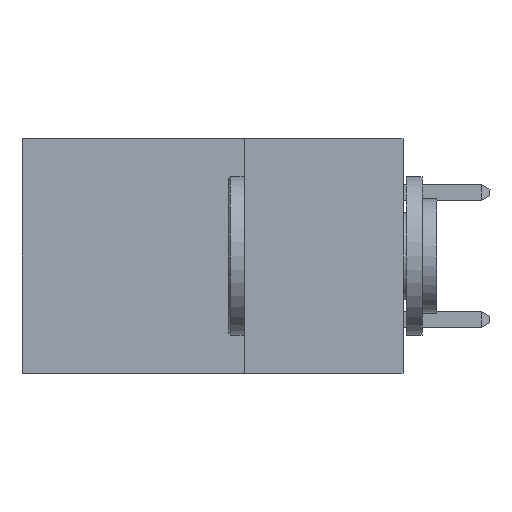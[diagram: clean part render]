
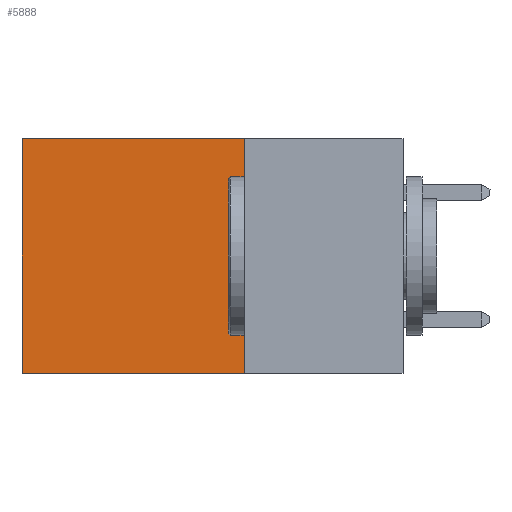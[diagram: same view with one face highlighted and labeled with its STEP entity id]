
A CAD part, left-side view. The second image highlights one B-rep face of the part: STEP entity #5888.
In plain terms, the highlighted planar face has unit normal (-1, 0, 0).
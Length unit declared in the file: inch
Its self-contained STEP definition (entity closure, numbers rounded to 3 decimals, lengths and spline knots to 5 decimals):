
#32 = VECTOR ( 'NONE', #170, 39.37008 ) ;
#118 = CARTESIAN_POINT ( 'NONE',  ( 0.2875, 0.25, -0.37 ) ) ;
#170 = DIRECTION ( 'NONE',  ( 0., 1., 0. ) ) ;
#578 = LINE ( 'NONE', #11281, #11457 ) ;
#1459 = EDGE_CURVE ( 'NONE', #9048, #6883, #3397, .T. ) ;
#2015 = EDGE_CURVE ( 'NONE', #9216, #11990, #4207, .T. ) ;
#2278 = DIRECTION ( 'NONE',  ( 1., 0., 0. ) ) ;
#2710 = ORIENTED_EDGE ( 'NONE', *, *, #3335, .F. ) ;
#3250 = CARTESIAN_POINT ( 'NONE',  ( 0.2875, 0.25, 0. ) ) ;
#3335 = EDGE_CURVE ( 'NONE', #11990, #6883, #11014, .T. ) ;
#3397 = LINE ( 'NONE', #9690, #5853 ) ;
#3884 = VECTOR ( 'NONE', #4990, 39.37008 ) ;
#4207 = LINE ( 'NONE', #5209, #3884 ) ;
#4990 = DIRECTION ( 'NONE',  ( 0., 0., -1. ) ) ;
#5109 = ORIENTED_EDGE ( 'NONE', *, *, #11385, .T. ) ;
#5135 = CARTESIAN_POINT ( 'NONE',  ( 0.2875, 0.6, -0.37 ) ) ;
#5209 = CARTESIAN_POINT ( 'NONE',  ( 0.2875, 0.25, 0. ) ) ;
#5252 = CARTESIAN_POINT ( 'NONE',  ( 0.2875, 0.6, 0. ) ) ;
#5508 = ORIENTED_EDGE ( 'NONE', *, *, #1459, .T. ) ;
#5853 = VECTOR ( 'NONE', #9373, 39.37008 ) ;
#5888 = ADVANCED_FACE ( 'NONE', ( #13067 ), #6490, .F. ) ;
#6490 = PLANE ( 'NONE',  #8403 ) ;
#6883 = VERTEX_POINT ( 'NONE', #5135 ) ;
#8403 = AXIS2_PLACEMENT_3D ( 'NONE', #13406, #2278, #9487 ) ;
#9048 = VERTEX_POINT ( 'NONE', #5252 ) ;
#9216 = VERTEX_POINT ( 'NONE', #3250 ) ;
#9373 = DIRECTION ( 'NONE',  ( 0., 0., -1. ) ) ;
#9487 = DIRECTION ( 'NONE',  ( 0., 0., -1. ) ) ;
#9690 = CARTESIAN_POINT ( 'NONE',  ( 0.2875, 0.6, 0. ) ) ;
#9985 = ORIENTED_EDGE ( 'NONE', *, *, #2015, .F. ) ;
#10312 = DIRECTION ( 'NONE',  ( 0., 1., 0. ) ) ;
#10817 = CARTESIAN_POINT ( 'NONE',  ( 0.2875, 0.25, -0.37 ) ) ;
#11014 = LINE ( 'NONE', #118, #32 ) ;
#11281 = CARTESIAN_POINT ( 'NONE',  ( 0.2875, 0.25, 0. ) ) ;
#11385 = EDGE_CURVE ( 'NONE', #9216, #9048, #578, .T. ) ;
#11457 = VECTOR ( 'NONE', #10312, 39.37008 ) ;
#11990 = VERTEX_POINT ( 'NONE', #10817 ) ;
#12778 = EDGE_LOOP ( 'NONE', ( #5508, #2710, #9985, #5109 ) ) ;
#13067 = FACE_OUTER_BOUND ( 'NONE', #12778, .T. ) ;
#13406 = CARTESIAN_POINT ( 'NONE',  ( 0.2875, 0.25, 0. ) ) ;
